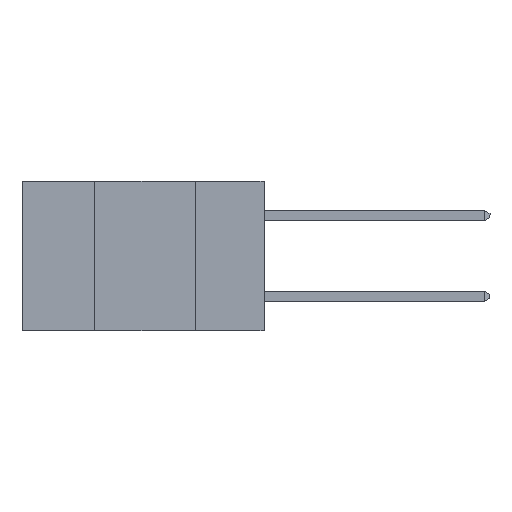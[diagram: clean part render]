
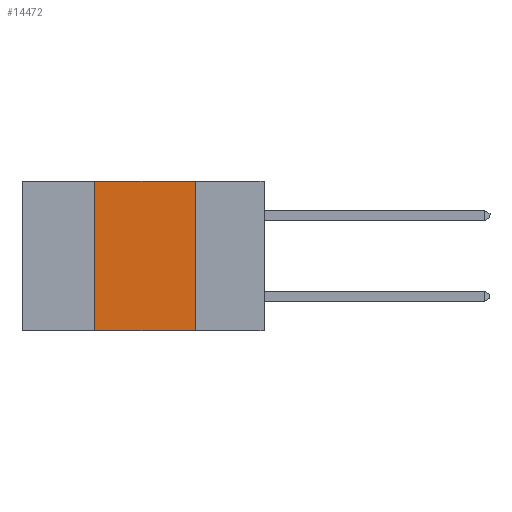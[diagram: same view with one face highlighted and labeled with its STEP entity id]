
A CAD part, left-side view. The second image highlights one B-rep face of the part: STEP entity #14472.
In plain terms, the highlighted planar face has unit normal (-1, 0, 0).
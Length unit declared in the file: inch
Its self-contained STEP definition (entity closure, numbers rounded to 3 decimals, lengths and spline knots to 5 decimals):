
#797 = EDGE_CURVE ( 'NONE', #15459, #6640, #12611, .T. ) ;
#1013 = ORIENTED_EDGE ( 'NONE', *, *, #4965, .F. ) ;
#1721 = DIRECTION ( 'NONE',  ( 0., 0., -1. ) ) ;
#2796 = EDGE_CURVE ( 'NONE', #15459, #18707, #5542, .T. ) ;
#3090 = CARTESIAN_POINT ( 'NONE',  ( 0., 0.42, 0. ) ) ;
#3382 = CARTESIAN_POINT ( 'NONE',  ( 0., 0.6, 0. ) ) ;
#3723 = CARTESIAN_POINT ( 'NONE',  ( 0., 0.17, 0. ) ) ;
#4087 = ORIENTED_EDGE ( 'NONE', *, *, #2796, .F. ) ;
#4123 = ORIENTED_EDGE ( 'NONE', *, *, #797, .T. ) ;
#4312 = CARTESIAN_POINT ( 'NONE',  ( 0., 0.6, -0.37 ) ) ;
#4379 = VECTOR ( 'NONE', #9500, 39.37008 ) ;
#4563 = VERTEX_POINT ( 'NONE', #3723 ) ;
#4965 = EDGE_CURVE ( 'NONE', #4563, #6640, #11271, .T. ) ;
#5334 = ORIENTED_EDGE ( 'NONE', *, *, #12893, .F. ) ;
#5542 = LINE ( 'NONE', #16670, #13255 ) ;
#6254 = VECTOR ( 'NONE', #14238, 39.37008 ) ;
#6370 = EDGE_LOOP ( 'NONE', ( #1013, #5334, #4087, #4123 ) ) ;
#6640 = VERTEX_POINT ( 'NONE', #9220 ) ;
#6705 = VECTOR ( 'NONE', #18269, 39.37008 ) ;
#7993 = PLANE ( 'NONE',  #17998 ) ;
#9220 = CARTESIAN_POINT ( 'NONE',  ( 0., 0.17, -0.37 ) ) ;
#9241 = DIRECTION ( 'NONE',  ( 0., 0., 1. ) ) ;
#9396 = LINE ( 'NONE', #3382, #6254 ) ;
#9500 = DIRECTION ( 'NONE',  ( 0., -1., 0. ) ) ;
#9586 = CARTESIAN_POINT ( 'NONE',  ( 0., 0.6, 0. ) ) ;
#11103 = DIRECTION ( 'NONE',  ( 1., 0., 0. ) ) ;
#11271 = LINE ( 'NONE', #18135, #6705 ) ;
#11800 = CARTESIAN_POINT ( 'NONE',  ( 0., 0.42, -0.37 ) ) ;
#12611 = LINE ( 'NONE', #4312, #4379 ) ;
#12893 = EDGE_CURVE ( 'NONE', #18707, #4563, #9396, .T. ) ;
#13149 = FACE_OUTER_BOUND ( 'NONE', #6370, .T. ) ;
#13255 = VECTOR ( 'NONE', #9241, 39.37008 ) ;
#14238 = DIRECTION ( 'NONE',  ( 0., -1., 0. ) ) ;
#14472 = ADVANCED_FACE ( 'NONE', ( #13149 ), #7993, .F. ) ;
#15459 = VERTEX_POINT ( 'NONE', #11800 ) ;
#16670 = CARTESIAN_POINT ( 'NONE',  ( 0., 0.42, 0. ) ) ;
#17998 = AXIS2_PLACEMENT_3D ( 'NONE', #9586, #11103, #1721 ) ;
#18135 = CARTESIAN_POINT ( 'NONE',  ( 0., 0.17, 0. ) ) ;
#18269 = DIRECTION ( 'NONE',  ( 0., 0., -1. ) ) ;
#18707 = VERTEX_POINT ( 'NONE', #3090 ) ;
